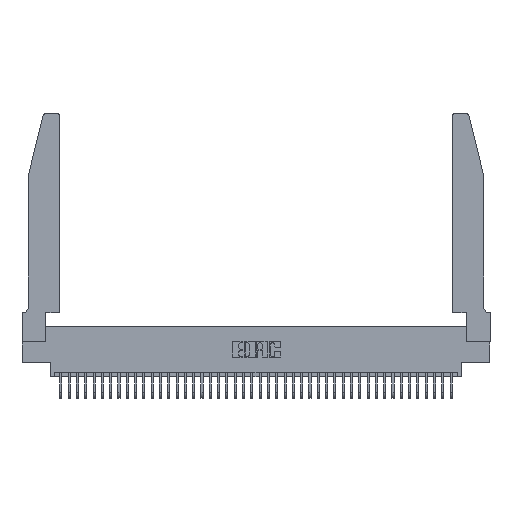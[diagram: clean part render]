
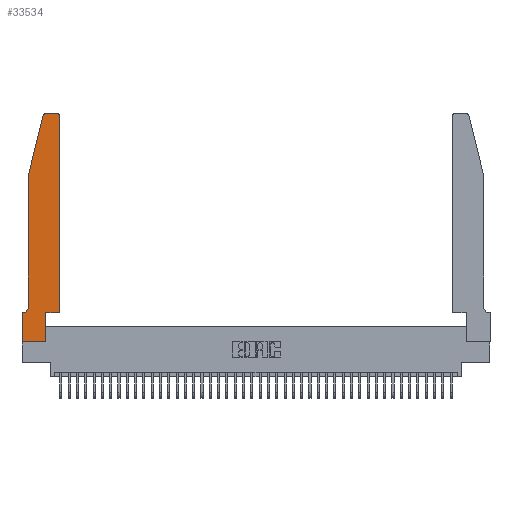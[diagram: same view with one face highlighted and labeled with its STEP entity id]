
A CAD part, top view. The second image highlights one B-rep face of the part: STEP entity #33534.
In plain terms, the highlighted planar face has unit normal (0, 0, 1).
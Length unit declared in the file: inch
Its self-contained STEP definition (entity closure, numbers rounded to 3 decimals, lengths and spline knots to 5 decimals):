
#219 = AXIS2_PLACEMENT_3D ( 'NONE', #17842, #11651, #33380 ) ;
#701 = DIRECTION ( 'NONE',  ( 0., -1., 0. ) ) ;
#907 = EDGE_CURVE ( 'NONE', #20067, #3657, #11310, .T. ) ;
#1072 = VERTEX_POINT ( 'NONE', #35343 ) ;
#1446 = VECTOR ( 'NONE', #36713, 39.37008 ) ;
#2310 = AXIS2_PLACEMENT_3D ( 'NONE', #16887, #38427, #20056 ) ;
#2325 = VECTOR ( 'NONE', #25856, 39.37008 ) ;
#2444 = LINE ( 'NONE', #5623, #1446 ) ;
#2876 = ORIENTED_EDGE ( 'NONE', *, *, #17580, .T. ) ;
#3657 = VERTEX_POINT ( 'NONE', #26625 ) ;
#4147 = CARTESIAN_POINT ( 'NONE',  ( 0.0755, 2., 0.37 ) ) ;
#4211 = VERTEX_POINT ( 'NONE', #26447 ) ;
#4716 = DIRECTION ( 'NONE',  ( 0., 0., 1. ) ) ;
#4842 = CARTESIAN_POINT ( 'NONE',  ( 0.25487, 2.72718, 0.37 ) ) ;
#5170 = CARTESIAN_POINT ( 'NONE',  ( 0.4205, 2.75, 0.37 ) ) ;
#5258 = DIRECTION ( 'NONE',  ( 1., 0., 0. ) ) ;
#5623 = CARTESIAN_POINT ( 'NONE',  ( 0.2865, 0.35, 0.37 ) ) ;
#5671 = AXIS2_PLACEMENT_3D ( 'NONE', #23517, #4716, #26653 ) ;
#6075 = CARTESIAN_POINT ( 'NONE',  ( 0.2865, 0.35, 0.37 ) ) ;
#6796 = ORIENTED_EDGE ( 'NONE', *, *, #9386, .T. ) ;
#7082 = EDGE_CURVE ( 'NONE', #10177, #20067, #37856, .T. ) ;
#7112 = VERTEX_POINT ( 'NONE', #4842 ) ;
#7293 = DIRECTION ( 'NONE',  ( -0.239, -0.971, 0. ) ) ;
#7959 = VERTEX_POINT ( 'NONE', #27392 ) ;
#8173 = VECTOR ( 'NONE', #7293, 39.37008 ) ;
#8203 = FACE_OUTER_BOUND ( 'NONE', #38500, .T. ) ;
#8296 = DIRECTION ( 'NONE',  ( 0., 0., -1. ) ) ;
#8482 = PLANE ( 'NONE',  #219 ) ;
#8561 = ORIENTED_EDGE ( 'NONE', *, *, #18207, .T. ) ;
#9386 = EDGE_CURVE ( 'NONE', #7112, #4211, #33009, .T. ) ;
#10075 = ORIENTED_EDGE ( 'NONE', *, *, #25472, .T. ) ;
#10177 = VERTEX_POINT ( 'NONE', #17429 ) ;
#10187 = CARTESIAN_POINT ( 'NONE',  ( 0.4505, 0.35, 0.37 ) ) ;
#10409 = ORIENTED_EDGE ( 'NONE', *, *, #19088, .T. ) ;
#11310 = LINE ( 'NONE', #34555, #34133 ) ;
#11337 = CARTESIAN_POINT ( 'NONE',  ( 0., 0., 0.37 ) ) ;
#11651 = DIRECTION ( 'NONE',  ( 0., 0., 1. ) ) ;
#11977 = VERTEX_POINT ( 'NONE', #11337 ) ;
#12995 = ORIENTED_EDGE ( 'NONE', *, *, #40084, .T. ) ;
#13269 = DIRECTION ( 'NONE',  ( 0., -1., 0. ) ) ;
#13681 = VERTEX_POINT ( 'NONE', #20008 ) ;
#15237 = VECTOR ( 'NONE', #23876, 39.37008 ) ;
#16123 = ORIENTED_EDGE ( 'NONE', *, *, #16239, .T. ) ;
#16239 = EDGE_CURVE ( 'NONE', #35010, #36608, #25109, .T. ) ;
#16495 = EDGE_CURVE ( 'NONE', #4211, #35010, #39847, .T. ) ;
#16887 = CARTESIAN_POINT ( 'NONE',  ( 0.284, 2.72, 0.37 ) ) ;
#17429 = CARTESIAN_POINT ( 'NONE',  ( 0.4505, 2.72, 0.37 ) ) ;
#17580 = EDGE_CURVE ( 'NONE', #11977, #7959, #39817, .T. ) ;
#17842 = CARTESIAN_POINT ( 'NONE',  ( 0., 0.35, 0.37 ) ) ;
#18207 = EDGE_CURVE ( 'NONE', #38577, #13681, #35016, .T. ) ;
#18822 = ORIENTED_EDGE ( 'NONE', *, *, #907, .T. ) ;
#19062 = VECTOR ( 'NONE', #19109, 39.37008 ) ;
#19088 = EDGE_CURVE ( 'NONE', #3657, #7112, #36831, .T. ) ;
#19109 = DIRECTION ( 'NONE',  ( -1., 0., 0. ) ) ;
#19205 = ORIENTED_EDGE ( 'NONE', *, *, #7082, .T. ) ;
#19217 = DIRECTION ( 'NONE',  ( -1., 0., 0. ) ) ;
#20008 = CARTESIAN_POINT ( 'NONE',  ( 0.4505, 0.35, 0.37 ) ) ;
#20056 = DIRECTION ( 'NONE',  ( 1., 0., 0. ) ) ;
#20067 = VERTEX_POINT ( 'NONE', #5170 ) ;
#20944 = CARTESIAN_POINT ( 'NONE',  ( 0.4505, 0.35, 0.37 ) ) ;
#22103 = CARTESIAN_POINT ( 'NONE',  ( 0.0755, 0.42, 0.37 ) ) ;
#22327 = EDGE_CURVE ( 'NONE', #1072, #11977, #29576, .T. ) ;
#22867 = CARTESIAN_POINT ( 'NONE',  ( 0., 0., 0.37 ) ) ;
#23517 = CARTESIAN_POINT ( 'NONE',  ( 0.4205, 2.72, 0.37 ) ) ;
#23876 = DIRECTION ( 'NONE',  ( 1., 0., 0. ) ) ;
#25058 = ORIENTED_EDGE ( 'NONE', *, *, #37377, .T. ) ;
#25109 = CIRCLE ( 'NONE', #31788, 0.07 ) ;
#25432 = LINE ( 'NONE', #37498, #19062 ) ;
#25472 = EDGE_CURVE ( 'NONE', #13681, #10177, #34498, .T. ) ;
#25856 = DIRECTION ( 'NONE',  ( 0., 1., 0. ) ) ;
#25974 = VECTOR ( 'NONE', #5258, 39.37008 ) ;
#26447 = CARTESIAN_POINT ( 'NONE',  ( 0.0755, 2., 0.37 ) ) ;
#26625 = CARTESIAN_POINT ( 'NONE',  ( 0.284, 2.75, 0.37 ) ) ;
#26653 = DIRECTION ( 'NONE',  ( 1., 0., 0. ) ) ;
#27078 = CARTESIAN_POINT ( 'NONE',  ( 0.0055, 0.42, 0.37 ) ) ;
#27392 = CARTESIAN_POINT ( 'NONE',  ( 0.2865, 0., 0.37 ) ) ;
#29576 = LINE ( 'NONE', #22867, #37605 ) ;
#30164 = DIRECTION ( 'NONE',  ( -1., 0., 0. ) ) ;
#31788 = AXIS2_PLACEMENT_3D ( 'NONE', #27078, #8296, #30164 ) ;
#33002 = CARTESIAN_POINT ( 'NONE',  ( 0.0055, 0.35, 0.37 ) ) ;
#33009 = LINE ( 'NONE', #4147, #8173 ) ;
#33380 = DIRECTION ( 'NONE',  ( 1., 0., 0. ) ) ;
#33534 = ADVANCED_FACE ( 'NONE', ( #8203 ), #8482, .T. ) ;
#34133 = VECTOR ( 'NONE', #19217, 39.37008 ) ;
#34429 = ORIENTED_EDGE ( 'NONE', *, *, #16495, .T. ) ;
#34498 = LINE ( 'NONE', #10187, #2325 ) ;
#34555 = CARTESIAN_POINT ( 'NONE',  ( 0.2605, 2.75, 0.37 ) ) ;
#35010 = VERTEX_POINT ( 'NONE', #22103 ) ;
#35016 = LINE ( 'NONE', #20944, #25974 ) ;
#35343 = CARTESIAN_POINT ( 'NONE',  ( 0., 0.35, 0.37 ) ) ;
#36018 = CARTESIAN_POINT ( 'NONE',  ( 0., 0., 0.37 ) ) ;
#36608 = VERTEX_POINT ( 'NONE', #33002 ) ;
#36713 = DIRECTION ( 'NONE',  ( 0., 1., 0. ) ) ;
#36831 = CIRCLE ( 'NONE', #2310, 0.03 ) ;
#37183 = ORIENTED_EDGE ( 'NONE', *, *, #22327, .T. ) ;
#37377 = EDGE_CURVE ( 'NONE', #7959, #38577, #2444, .T. ) ;
#37498 = CARTESIAN_POINT ( 'NONE',  ( 0.0755, 0.35, 0.37 ) ) ;
#37605 = VECTOR ( 'NONE', #701, 39.37008 ) ;
#37856 = CIRCLE ( 'NONE', #5671, 0.03 ) ;
#37955 = CARTESIAN_POINT ( 'NONE',  ( 0.0755, 2., 0.37 ) ) ;
#38427 = DIRECTION ( 'NONE',  ( 0., 0., 1. ) ) ;
#38500 = EDGE_LOOP ( 'NONE', ( #18822, #10409, #6796, #34429, #16123, #12995, #37183, #2876, #25058, #8561, #10075, #19205 ) ) ;
#38577 = VERTEX_POINT ( 'NONE', #6075 ) ;
#38886 = VECTOR ( 'NONE', #13269, 39.37008 ) ;
#39817 = LINE ( 'NONE', #36018, #15237 ) ;
#39847 = LINE ( 'NONE', #37955, #38886 ) ;
#40084 = EDGE_CURVE ( 'NONE', #36608, #1072, #25432, .T. ) ;
